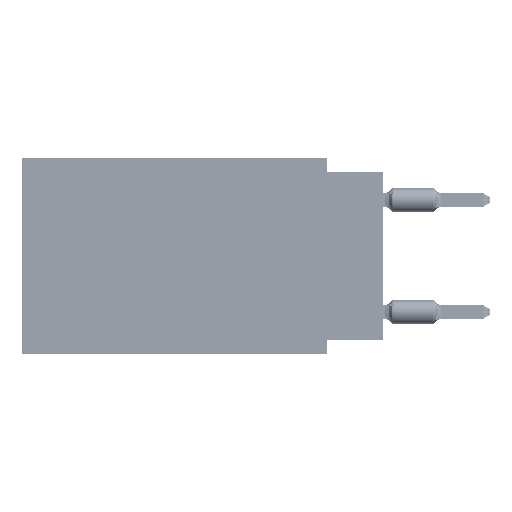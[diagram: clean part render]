
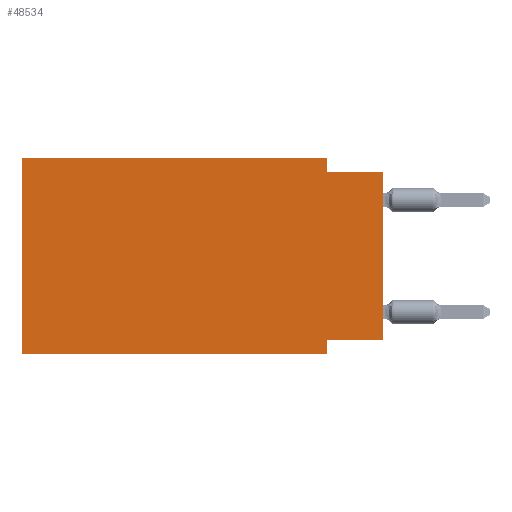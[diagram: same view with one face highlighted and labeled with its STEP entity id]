
A CAD part, left-side view. The second image highlights one B-rep face of the part: STEP entity #48534.
In plain terms, the highlighted planar face has unit normal (-1, 0, 0).
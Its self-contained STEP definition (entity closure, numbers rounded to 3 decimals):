
#1275 = EDGE_CURVE ( 'NONE', #44245, #32955, #90982, .T. ) ;
#2522 = LINE ( 'NONE', #71436, #78785 ) ;
#2836 = DIRECTION ( 'NONE',  ( 0., -1., 0. ) ) ;
#2919 = EDGE_CURVE ( 'NONE', #70384, #44245, #24807, .T. ) ;
#3879 = CARTESIAN_POINT ( 'NONE',  ( 0., 0., -8.255 ) ) ;
#5832 = CARTESIAN_POINT ( 'NONE',  ( 0., 16.383, -8.89 ) ) ;
#12008 = AXIS2_PLACEMENT_3D ( 'NONE', #24304, #42809, #110145 ) ;
#12054 = EDGE_CURVE ( 'NONE', #75071, #32955, #92617, .T. ) ;
#12104 = DIRECTION ( 'NONE',  ( 0., 0., 1. ) ) ;
#17458 = VECTOR ( 'NONE', #29575, 1000. ) ;
#18824 = CARTESIAN_POINT ( 'NONE',  ( 0., 2.54, 0. ) ) ;
#23597 = DIRECTION ( 'NONE',  ( 0., 1., 0. ) ) ;
#24304 = CARTESIAN_POINT ( 'NONE',  ( 0., 16.383, 0. ) ) ;
#24807 = LINE ( 'NONE', #3879, #83487 ) ;
#24831 = CARTESIAN_POINT ( 'NONE',  ( 0., 2.54, -8.89 ) ) ;
#24922 = CARTESIAN_POINT ( 'NONE',  ( 0., 2.54, -8.89 ) ) ;
#26556 = CARTESIAN_POINT ( 'NONE',  ( 0., 16.383, 0. ) ) ;
#28845 = ORIENTED_EDGE ( 'NONE', *, *, #12054, .T. ) ;
#29575 = DIRECTION ( 'NONE',  ( 0., -1., 0. ) ) ;
#30478 = EDGE_CURVE ( 'NONE', #90288, #54353, #44451, .T. ) ;
#31852 = VECTOR ( 'NONE', #62571, 1000. ) ;
#32011 = EDGE_CURVE ( 'NONE', #75071, #90288, #2522, .T. ) ;
#32420 = CARTESIAN_POINT ( 'NONE',  ( 0., 0., -0.635 ) ) ;
#32955 = VERTEX_POINT ( 'NONE', #24831 ) ;
#33320 = ORIENTED_EDGE ( 'NONE', *, *, #59775, .F. ) ;
#34471 = ORIENTED_EDGE ( 'NONE', *, *, #108636, .F. ) ;
#35202 = DIRECTION ( 'NONE',  ( 0., -1., 0. ) ) ;
#37948 = DIRECTION ( 'NONE',  ( 0., 0., -1. ) ) ;
#42497 = VECTOR ( 'NONE', #12104, 1000. ) ;
#42809 = DIRECTION ( 'NONE',  ( 1., 0., 0. ) ) ;
#44163 = VECTOR ( 'NONE', #37948, 1000. ) ;
#44245 = VERTEX_POINT ( 'NONE', #109198 ) ;
#44451 = LINE ( 'NONE', #26556, #100235 ) ;
#46879 = CARTESIAN_POINT ( 'NONE',  ( 0., 16.383, -8.89 ) ) ;
#47814 = LINE ( 'NONE', #18824, #44163 ) ;
#48534 = ADVANCED_FACE ( 'NONE', ( #101470 ), #79875, .F. ) ;
#48885 = CARTESIAN_POINT ( 'NONE',  ( 0., 0., -8.255 ) ) ;
#49406 = DIRECTION ( 'NONE',  ( 0., 0., 1. ) ) ;
#49879 = CARTESIAN_POINT ( 'NONE',  ( 0., 2.54, 0. ) ) ;
#50323 = LINE ( 'NONE', #68255, #42497 ) ;
#54353 = VERTEX_POINT ( 'NONE', #49879 ) ;
#59716 = EDGE_CURVE ( 'NONE', #70384, #106399, #50323, .T. ) ;
#59775 = EDGE_CURVE ( 'NONE', #70563, #106399, #115846, .T. ) ;
#62571 = DIRECTION ( 'NONE',  ( 0., 0., -1. ) ) ;
#68255 = CARTESIAN_POINT ( 'NONE',  ( 0., 0., 0. ) ) ;
#69861 = CARTESIAN_POINT ( 'NONE',  ( 0., 2.54, -0.635 ) ) ;
#70384 = VERTEX_POINT ( 'NONE', #48885 ) ;
#70563 = VERTEX_POINT ( 'NONE', #69861 ) ;
#71339 = CARTESIAN_POINT ( 'NONE',  ( 0., 0., -0.635 ) ) ;
#71436 = CARTESIAN_POINT ( 'NONE',  ( 0., 16.383, 0. ) ) ;
#75071 = VERTEX_POINT ( 'NONE', #5832 ) ;
#78423 = ORIENTED_EDGE ( 'NONE', *, *, #1275, .F. ) ;
#78785 = VECTOR ( 'NONE', #49406, 1000. ) ;
#79415 = CARTESIAN_POINT ( 'NONE',  ( 0., 16.383, 0. ) ) ;
#79875 = PLANE ( 'NONE',  #12008 ) ;
#83487 = VECTOR ( 'NONE', #23597, 1000. ) ;
#90288 = VERTEX_POINT ( 'NONE', #79415 ) ;
#90982 = LINE ( 'NONE', #24922, #31852 ) ;
#91343 = EDGE_LOOP ( 'NONE', ( #101021, #33320, #34471, #100160, #108182, #28845, #78423, #122056 ) ) ;
#92617 = LINE ( 'NONE', #46879, #17458 ) ;
#100160 = ORIENTED_EDGE ( 'NONE', *, *, #30478, .F. ) ;
#100235 = VECTOR ( 'NONE', #35202, 1000. ) ;
#101021 = ORIENTED_EDGE ( 'NONE', *, *, #59716, .T. ) ;
#101470 = FACE_OUTER_BOUND ( 'NONE', #91343, .T. ) ;
#106399 = VERTEX_POINT ( 'NONE', #71339 ) ;
#108182 = ORIENTED_EDGE ( 'NONE', *, *, #32011, .F. ) ;
#108636 = EDGE_CURVE ( 'NONE', #54353, #70563, #47814, .T. ) ;
#109198 = CARTESIAN_POINT ( 'NONE',  ( 0., 2.54, -8.255 ) ) ;
#110145 = DIRECTION ( 'NONE',  ( 0., 0., -1. ) ) ;
#115846 = LINE ( 'NONE', #32420, #117492 ) ;
#117492 = VECTOR ( 'NONE', #2836, 1000. ) ;
#122056 = ORIENTED_EDGE ( 'NONE', *, *, #2919, .F. ) ;
